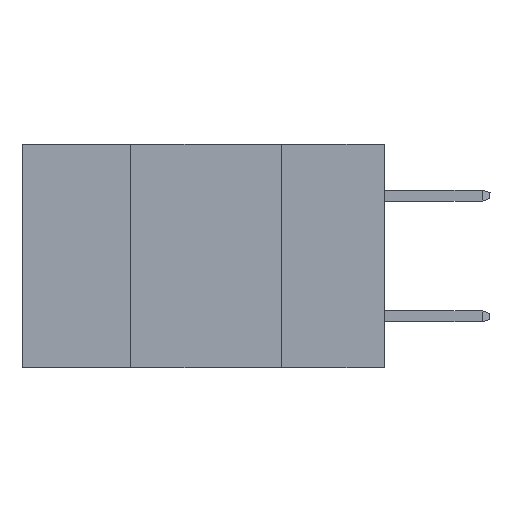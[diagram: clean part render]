
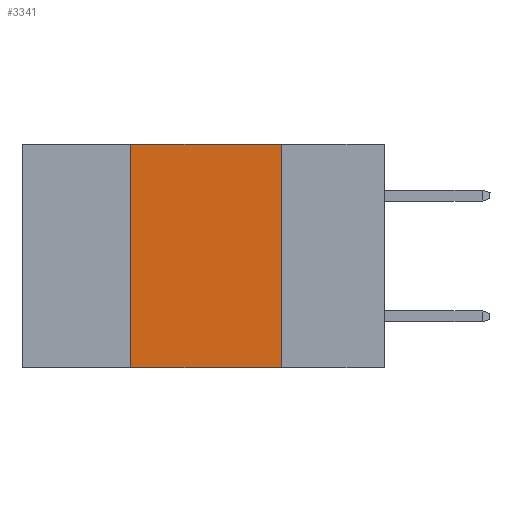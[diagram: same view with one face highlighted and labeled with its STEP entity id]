
A CAD part, left-side view. The second image highlights one B-rep face of the part: STEP entity #3341.
In plain terms, the highlighted planar face has unit normal (-1, 0, 0).
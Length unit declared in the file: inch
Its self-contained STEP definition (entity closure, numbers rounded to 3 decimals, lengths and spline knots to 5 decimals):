
#473 = CARTESIAN_POINT ( 'NONE',  ( 0., 0.6, 0. ) ) ;
#491 = VERTEX_POINT ( 'NONE', #21588 ) ;
#1206 = EDGE_CURVE ( 'NONE', #12356, #19250, #12321, .T. ) ;
#1314 = ORIENTED_EDGE ( 'NONE', *, *, #8441, .F. ) ;
#1640 = VERTEX_POINT ( 'NONE', #16627 ) ;
#3104 = ORIENTED_EDGE ( 'NONE', *, *, #10890, .F. ) ;
#3270 = VECTOR ( 'NONE', #16149, 39.37008 ) ;
#3341 = ADVANCED_FACE ( 'NONE', ( #8859 ), #19039, .F. ) ;
#4088 = DIRECTION ( 'NONE',  ( 0., 0., -1. ) ) ;
#5727 = DIRECTION ( 'NONE',  ( 0., 0., 1. ) ) ;
#6470 = EDGE_CURVE ( 'NONE', #1640, #491, #21957, .T. ) ;
#7079 = LINE ( 'NONE', #16324, #10741 ) ;
#8009 = ORIENTED_EDGE ( 'NONE', *, *, #6470, .T. ) ;
#8441 = EDGE_CURVE ( 'NONE', #1640, #12356, #20986, .T. ) ;
#8859 = FACE_OUTER_BOUND ( 'NONE', #16417, .T. ) ;
#10122 = DIRECTION ( 'NONE',  ( 1., 0., 0. ) ) ;
#10741 = VECTOR ( 'NONE', #4088, 39.37008 ) ;
#10890 = EDGE_CURVE ( 'NONE', #19250, #491, #7079, .T. ) ;
#12048 = CARTESIAN_POINT ( 'NONE',  ( 0., 0.6, -0.37 ) ) ;
#12152 = CARTESIAN_POINT ( 'NONE',  ( 0., 0.6, 0. ) ) ;
#12321 = LINE ( 'NONE', #473, #3270 ) ;
#12356 = VERTEX_POINT ( 'NONE', #20595 ) ;
#13780 = ORIENTED_EDGE ( 'NONE', *, *, #1206, .F. ) ;
#14729 = CARTESIAN_POINT ( 'NONE',  ( 0., 0.42, 0. ) ) ;
#16149 = DIRECTION ( 'NONE',  ( 0., -1., 0. ) ) ;
#16324 = CARTESIAN_POINT ( 'NONE',  ( 0., 0.17, 0. ) ) ;
#16417 = EDGE_LOOP ( 'NONE', ( #3104, #13780, #1314, #8009 ) ) ;
#16627 = CARTESIAN_POINT ( 'NONE',  ( 0., 0.42, -0.37 ) ) ;
#18618 = AXIS2_PLACEMENT_3D ( 'NONE', #12152, #10122, #20827 ) ;
#19039 = PLANE ( 'NONE',  #18618 ) ;
#19250 = VERTEX_POINT ( 'NONE', #20805 ) ;
#20595 = CARTESIAN_POINT ( 'NONE',  ( 0., 0.42, 0. ) ) ;
#20788 = DIRECTION ( 'NONE',  ( 0., -1., 0. ) ) ;
#20805 = CARTESIAN_POINT ( 'NONE',  ( 0., 0.17, 0. ) ) ;
#20827 = DIRECTION ( 'NONE',  ( 0., 0., -1. ) ) ;
#20986 = LINE ( 'NONE', #14729, #22370 ) ;
#21395 = VECTOR ( 'NONE', #20788, 39.37008 ) ;
#21588 = CARTESIAN_POINT ( 'NONE',  ( 0., 0.17, -0.37 ) ) ;
#21957 = LINE ( 'NONE', #12048, #21395 ) ;
#22370 = VECTOR ( 'NONE', #5727, 39.37008 ) ;
